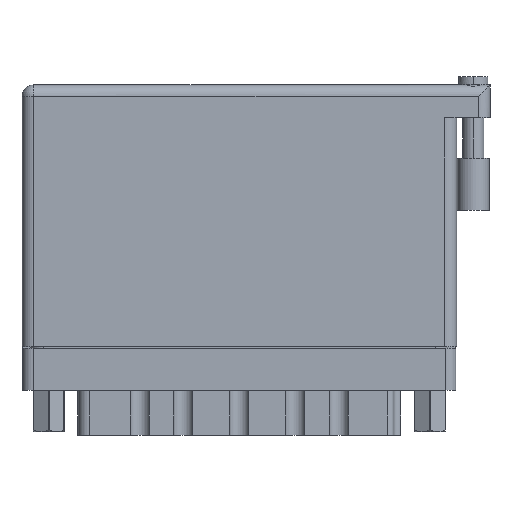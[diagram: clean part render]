
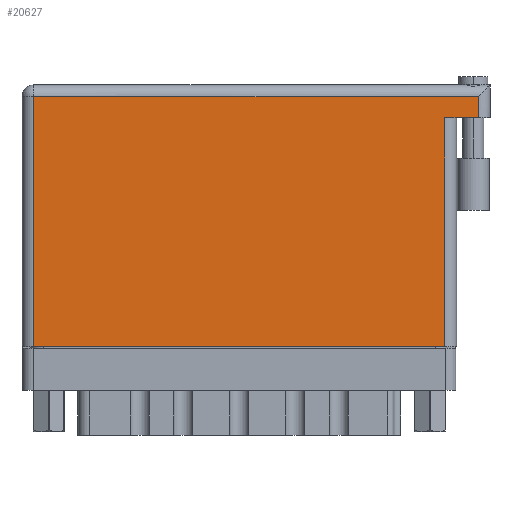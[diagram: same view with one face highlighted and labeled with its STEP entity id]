
A CAD part, front view. The second image highlights one B-rep face of the part: STEP entity #20627.
In plain terms, the highlighted face is planar.
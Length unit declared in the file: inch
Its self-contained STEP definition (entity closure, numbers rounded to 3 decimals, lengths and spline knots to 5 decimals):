
#395 = CARTESIAN_POINT ( 'NONE',  ( 0., 0., 0. ) ) ;
#455 = CARTESIAN_POINT ( 'NONE',  ( 2.8, 1.369, 0. ) ) ;
#1087 = DIRECTION ( 'NONE',  ( -1., 0., 0. ) ) ;
#1978 = FACE_OUTER_BOUND ( 'NONE', #41733, .T. ) ;
#2716 = CARTESIAN_POINT ( 'NONE',  ( 0.07, 1.496, 0. ) ) ;
#3443 = VECTOR ( 'NONE', #31047, 39.37008 ) ;
#4336 = DIRECTION ( 'NONE',  ( 0., 0., -1. ) ) ;
#5710 = LINE ( 'NONE', #37925, #58860 ) ;
#6617 = VERTEX_POINT ( 'NONE', #35281 ) ;
#10369 = VERTEX_POINT ( 'NONE', #13064 ) ;
#10396 = LINE ( 'NONE', #30765, #31276 ) ;
#11969 = VERTEX_POINT ( 'NONE', #27377 ) ;
#12357 = EDGE_CURVE ( 'NONE', #16324, #6617, #5710, .T. ) ;
#13064 = CARTESIAN_POINT ( 'NONE',  ( 2.73, 1.496, 0. ) ) ;
#14238 = ORIENTED_EDGE ( 'NONE', *, *, #26221, .T. ) ;
#15161 = VECTOR ( 'NONE', #1087, 39.37008 ) ;
#16017 = DIRECTION ( 'NONE',  ( 0., 1., 0. ) ) ;
#16324 = VERTEX_POINT ( 'NONE', #2716 ) ;
#17853 = EDGE_CURVE ( 'NONE', #11969, #40878, #27866, .T. ) ;
#20627 = ADVANCED_FACE ( 'NONE', ( #1978 ), #56851, .F. ) ;
#22117 = AXIS2_PLACEMENT_3D ( 'NONE', #62052, #4336, #56656 ) ;
#23669 = LINE ( 'NONE', #395, #61875 ) ;
#24160 = EDGE_CURVE ( 'NONE', #11969, #10369, #37602, .T. ) ;
#26056 = CARTESIAN_POINT ( 'NONE',  ( 2.73, 1.566, 0. ) ) ;
#26221 = EDGE_CURVE ( 'NONE', #6617, #27204, #23669, .T. ) ;
#27204 = VERTEX_POINT ( 'NONE', #29897 ) ;
#27377 = CARTESIAN_POINT ( 'NONE',  ( 2.73, 1.369, 0. ) ) ;
#27866 = LINE ( 'NONE', #455, #15161 ) ;
#29897 = CARTESIAN_POINT ( 'NONE',  ( 2.53, 0., 0. ) ) ;
#30765 = CARTESIAN_POINT ( 'NONE',  ( 2.53, 1.369, 0. ) ) ;
#31047 = DIRECTION ( 'NONE',  ( -1., 0., 0. ) ) ;
#31276 = VECTOR ( 'NONE', #16017, 39.37008 ) ;
#33426 = ORIENTED_EDGE ( 'NONE', *, *, #42979, .T. ) ;
#33615 = ORIENTED_EDGE ( 'NONE', *, *, #17853, .F. ) ;
#34027 = DIRECTION ( 'NONE',  ( 1., 0., 0. ) ) ;
#34197 = EDGE_CURVE ( 'NONE', #10369, #16324, #37863, .T. ) ;
#35281 = CARTESIAN_POINT ( 'NONE',  ( 0.07, 0., 0. ) ) ;
#35671 = DIRECTION ( 'NONE',  ( 0., 1., 0. ) ) ;
#36069 = CARTESIAN_POINT ( 'NONE',  ( 0., 1.496, 0. ) ) ;
#37602 = LINE ( 'NONE', #26056, #60064 ) ;
#37863 = LINE ( 'NONE', #36069, #3443 ) ;
#37925 = CARTESIAN_POINT ( 'NONE',  ( 0.07, 0., 0. ) ) ;
#40878 = VERTEX_POINT ( 'NONE', #48058 ) ;
#41733 = EDGE_LOOP ( 'NONE', ( #14238, #33426, #33615, #43766, #48628, #48826 ) ) ;
#42979 = EDGE_CURVE ( 'NONE', #27204, #40878, #10396, .T. ) ;
#43766 = ORIENTED_EDGE ( 'NONE', *, *, #24160, .T. ) ;
#48058 = CARTESIAN_POINT ( 'NONE',  ( 2.53, 1.369, 0. ) ) ;
#48628 = ORIENTED_EDGE ( 'NONE', *, *, #34197, .T. ) ;
#48826 = ORIENTED_EDGE ( 'NONE', *, *, #12357, .T. ) ;
#56656 = DIRECTION ( 'NONE',  ( -1., 0., 0. ) ) ;
#56810 = DIRECTION ( 'NONE',  ( 0., -1., 0. ) ) ;
#56851 = PLANE ( 'NONE',  #22117 ) ;
#58860 = VECTOR ( 'NONE', #56810, 39.37008 ) ;
#60064 = VECTOR ( 'NONE', #35671, 39.37008 ) ;
#61875 = VECTOR ( 'NONE', #34027, 39.37008 ) ;
#62052 = CARTESIAN_POINT ( 'NONE',  ( 0., 1.566, 0. ) ) ;
